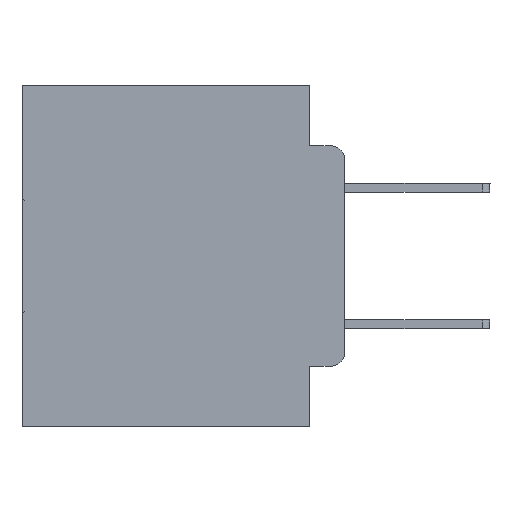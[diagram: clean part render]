
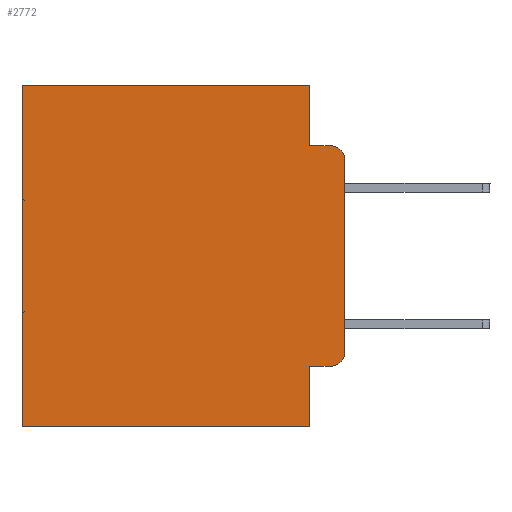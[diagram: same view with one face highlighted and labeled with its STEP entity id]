
A CAD part, left-side view. The second image highlights one B-rep face of the part: STEP entity #2772.
In plain terms, the highlighted planar face has unit normal (-1, 0, 0).
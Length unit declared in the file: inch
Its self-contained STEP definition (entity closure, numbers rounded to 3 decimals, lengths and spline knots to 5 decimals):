
#268 = CARTESIAN_POINT ( 'NONE',  ( 0.298, 0.473, 0. ) ) ;
#460 = LINE ( 'NONE', #30718, #19620 ) ;
#744 = CARTESIAN_POINT ( 'NONE',  ( 0.298, 0.051, 0. ) ) ;
#1054 = LINE ( 'NONE', #744, #13226 ) ;
#1132 = CIRCLE ( 'NONE', #22109, 0.02 ) ;
#1942 = EDGE_CURVE ( 'NONE', #28981, #21888, #9259, .T. ) ;
#1987 = LINE ( 'NONE', #9735, #16809 ) ;
#2329 = CARTESIAN_POINT ( 'NONE',  ( 0.298, 0.051, -0.0885 ) ) ;
#2470 = ORIENTED_EDGE ( 'NONE', *, *, #10903, .F. ) ;
#2772 = ADVANCED_FACE ( 'NONE', ( #27138 ), #9363, .F. ) ;
#3412 = CARTESIAN_POINT ( 'NONE',  ( 0.298, 0.473, -0.5 ) ) ;
#3744 = EDGE_CURVE ( 'NONE', #29981, #30018, #460, .T. ) ;
#3966 = VERTEX_POINT ( 'NONE', #21486 ) ;
#4762 = CARTESIAN_POINT ( 'NONE',  ( 0.298, 0.051, -0.4115 ) ) ;
#5683 = LINE ( 'NONE', #268, #19339 ) ;
#5714 = LINE ( 'NONE', #28096, #13650 ) ;
#7486 = EDGE_CURVE ( 'NONE', #20527, #23170, #1132, .T. ) ;
#7652 = EDGE_CURVE ( 'NONE', #28981, #3966, #1054, .T. ) ;
#8978 = ORIENTED_EDGE ( 'NONE', *, *, #15870, .F. ) ;
#9217 = DIRECTION ( 'NONE',  ( 0., 0., -1. ) ) ;
#9259 = LINE ( 'NONE', #16966, #29664 ) ;
#9363 = PLANE ( 'NONE',  #22143 ) ;
#9735 = CARTESIAN_POINT ( 'NONE',  ( 0.298, 0., -0.5 ) ) ;
#9896 = CARTESIAN_POINT ( 'NONE',  ( 0.298, 0.051, 0. ) ) ;
#9990 = DIRECTION ( 'NONE',  ( -1., 0., 0. ) ) ;
#10330 = CARTESIAN_POINT ( 'NONE',  ( 0.298, 0.02, -0.3915 ) ) ;
#10903 = EDGE_CURVE ( 'NONE', #30018, #23170, #15528, .T. ) ;
#11116 = DIRECTION ( 'NONE',  ( 0., 0., -1. ) ) ;
#11278 = CARTESIAN_POINT ( 'NONE',  ( 0.298, 0.051, -0.0885 ) ) ;
#11742 = DIRECTION ( 'NONE',  ( 0., -1., 0. ) ) ;
#11826 = VECTOR ( 'NONE', #26670, 39.37008 ) ;
#12400 = VERTEX_POINT ( 'NONE', #30835 ) ;
#13010 = EDGE_CURVE ( 'NONE', #29981, #18796, #21563, .T. ) ;
#13226 = VECTOR ( 'NONE', #11116, 39.37008 ) ;
#13650 = VECTOR ( 'NONE', #15576, 39.37008 ) ;
#14594 = ORIENTED_EDGE ( 'NONE', *, *, #27100, .T. ) ;
#14798 = EDGE_CURVE ( 'NONE', #18796, #30529, #5683, .T. ) ;
#15037 = ORIENTED_EDGE ( 'NONE', *, *, #7652, .F. ) ;
#15046 = CARTESIAN_POINT ( 'NONE',  ( 0.298, 0.02, -0.1085 ) ) ;
#15528 = LINE ( 'NONE', #11278, #18031 ) ;
#15576 = DIRECTION ( 'NONE',  ( 0., 0., -1. ) ) ;
#15673 = DIRECTION ( 'NONE',  ( 0., -1., 0. ) ) ;
#15695 = DIRECTION ( 'NONE',  ( 0., 0., -1. ) ) ;
#15749 = EDGE_LOOP ( 'NONE', ( #8978, #26163, #2470, #17586, #21016, #26835, #26041, #15037, #16901, #14594 ) ) ;
#15870 = EDGE_CURVE ( 'NONE', #20527, #12400, #5714, .T. ) ;
#16809 = VECTOR ( 'NONE', #24197, 39.37008 ) ;
#16901 = ORIENTED_EDGE ( 'NONE', *, *, #1942, .T. ) ;
#16966 = CARTESIAN_POINT ( 'NONE',  ( 0.298, 0.051, -0.4115 ) ) ;
#17237 = DIRECTION ( 'NONE',  ( 1., 0., 0. ) ) ;
#17586 = ORIENTED_EDGE ( 'NONE', *, *, #3744, .F. ) ;
#17667 = DIRECTION ( 'NONE',  ( -1., 0., 0. ) ) ;
#18031 = VECTOR ( 'NONE', #15673, 39.37008 ) ;
#18355 = AXIS2_PLACEMENT_3D ( 'NONE', #10330, #9990, #20340 ) ;
#18376 = DIRECTION ( 'NONE',  ( 0., 0., -1. ) ) ;
#18796 = VERTEX_POINT ( 'NONE', #31307 ) ;
#19036 = CARTESIAN_POINT ( 'NONE',  ( 0.298, 0., -0.1085 ) ) ;
#19339 = VECTOR ( 'NONE', #15695, 39.37008 ) ;
#19620 = VECTOR ( 'NONE', #18376, 39.37008 ) ;
#19907 = CIRCLE ( 'NONE', #18355, 0.02 ) ;
#20310 = DIRECTION ( 'NONE',  ( 0., 0., -1. ) ) ;
#20340 = DIRECTION ( 'NONE',  ( 0., 0., -1. ) ) ;
#20527 = VERTEX_POINT ( 'NONE', #19036 ) ;
#21016 = ORIENTED_EDGE ( 'NONE', *, *, #13010, .T. ) ;
#21343 = CARTESIAN_POINT ( 'NONE',  ( 0.298, 0.02, -0.4115 ) ) ;
#21486 = CARTESIAN_POINT ( 'NONE',  ( 0.298, 0.051, -0.5 ) ) ;
#21563 = LINE ( 'NONE', #23890, #11826 ) ;
#21888 = VERTEX_POINT ( 'NONE', #21343 ) ;
#22109 = AXIS2_PLACEMENT_3D ( 'NONE', #15046, #17667, #20310 ) ;
#22143 = AXIS2_PLACEMENT_3D ( 'NONE', #32207, #17237, #9217 ) ;
#23170 = VERTEX_POINT ( 'NONE', #23522 ) ;
#23522 = CARTESIAN_POINT ( 'NONE',  ( 0.298, 0.02, -0.0885 ) ) ;
#23890 = CARTESIAN_POINT ( 'NONE',  ( 0.298, 0., 0. ) ) ;
#24197 = DIRECTION ( 'NONE',  ( 0., 1., 0. ) ) ;
#26041 = ORIENTED_EDGE ( 'NONE', *, *, #30003, .F. ) ;
#26163 = ORIENTED_EDGE ( 'NONE', *, *, #7486, .T. ) ;
#26670 = DIRECTION ( 'NONE',  ( 0., 1., 0. ) ) ;
#26835 = ORIENTED_EDGE ( 'NONE', *, *, #14798, .T. ) ;
#27100 = EDGE_CURVE ( 'NONE', #21888, #12400, #19907, .T. ) ;
#27138 = FACE_OUTER_BOUND ( 'NONE', #15749, .T. ) ;
#28096 = CARTESIAN_POINT ( 'NONE',  ( 0.298, 0., 0. ) ) ;
#28981 = VERTEX_POINT ( 'NONE', #4762 ) ;
#29664 = VECTOR ( 'NONE', #11742, 39.37008 ) ;
#29981 = VERTEX_POINT ( 'NONE', #9896 ) ;
#30003 = EDGE_CURVE ( 'NONE', #3966, #30529, #1987, .T. ) ;
#30018 = VERTEX_POINT ( 'NONE', #2329 ) ;
#30529 = VERTEX_POINT ( 'NONE', #3412 ) ;
#30718 = CARTESIAN_POINT ( 'NONE',  ( 0.298, 0.051, 0. ) ) ;
#30835 = CARTESIAN_POINT ( 'NONE',  ( 0.298, 0., -0.3915 ) ) ;
#31307 = CARTESIAN_POINT ( 'NONE',  ( 0.298, 0.473, 0. ) ) ;
#32207 = CARTESIAN_POINT ( 'NONE',  ( 0.298, 0., 0. ) ) ;
